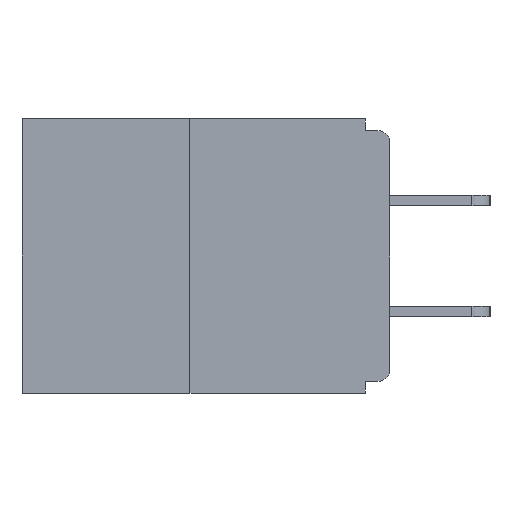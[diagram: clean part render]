
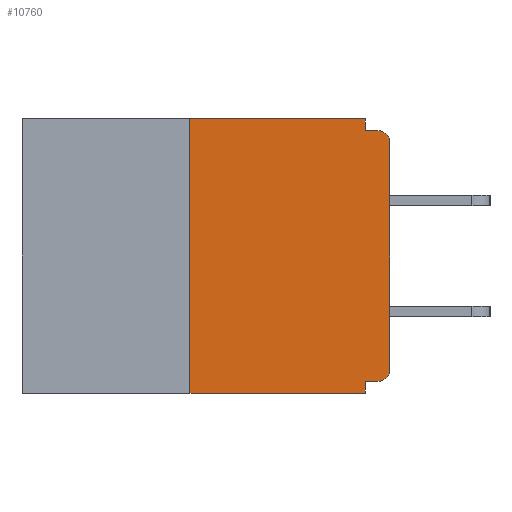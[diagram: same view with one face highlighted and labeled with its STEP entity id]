
A CAD part, left-side view. The second image highlights one B-rep face of the part: STEP entity #10760.
In plain terms, the highlighted planar face has unit normal (-1, 0, 0).
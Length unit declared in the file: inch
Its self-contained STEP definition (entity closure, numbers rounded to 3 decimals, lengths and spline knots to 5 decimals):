
#890 = LINE ( 'NONE', #17852, #12626 ) ;
#1479 = FACE_OUTER_BOUND ( 'NONE', #20674, .T. ) ;
#1658 = EDGE_CURVE ( 'NONE', #22780, #31343, #8278, .T. ) ;
#1729 = DIRECTION ( 'NONE',  ( 0., 0., -1. ) ) ;
#1784 = CARTESIAN_POINT ( 'NONE',  ( 0., 0.031, 0. ) ) ;
#2035 = DIRECTION ( 'NONE',  ( 0., 0., -1. ) ) ;
#2279 = AXIS2_PLACEMENT_3D ( 'NONE', #23241, #10829, #30538 ) ;
#2315 = VECTOR ( 'NONE', #21846, 39.37008 ) ;
#2624 = CARTESIAN_POINT ( 'NONE',  ( 0., 0.46, -0.343 ) ) ;
#2705 = CARTESIAN_POINT ( 'NONE',  ( 0., 0., -0.03 ) ) ;
#3207 = EDGE_CURVE ( 'NONE', #7098, #22780, #890, .T. ) ;
#3478 = LINE ( 'NONE', #25552, #4742 ) ;
#4213 = ORIENTED_EDGE ( 'NONE', *, *, #1658, .F. ) ;
#4228 = CARTESIAN_POINT ( 'NONE',  ( 0., 0.015, -0.03 ) ) ;
#4742 = VECTOR ( 'NONE', #1729, 39.37008 ) ;
#4753 = ORIENTED_EDGE ( 'NONE', *, *, #20375, .T. ) ;
#5220 = CARTESIAN_POINT ( 'NONE',  ( 0., 0.25, 0. ) ) ;
#5542 = CIRCLE ( 'NONE', #27365, 0.015 ) ;
#5695 = VECTOR ( 'NONE', #2035, 39.37008 ) ;
#6426 = DIRECTION ( 'NONE',  ( 0., 0., -1. ) ) ;
#6521 = CARTESIAN_POINT ( 'NONE',  ( 0., 0., -0.328 ) ) ;
#6990 = EDGE_CURVE ( 'NONE', #10298, #8557, #23359, .T. ) ;
#7098 = VERTEX_POINT ( 'NONE', #5220 ) ;
#7487 = EDGE_CURVE ( 'NONE', #10595, #27590, #17248, .T. ) ;
#7835 = CARTESIAN_POINT ( 'NONE',  ( 0., 0., -0.313 ) ) ;
#8038 = DIRECTION ( 'NONE',  ( 0., -1., 0. ) ) ;
#8278 = LINE ( 'NONE', #28575, #5695 ) ;
#8441 = VECTOR ( 'NONE', #30998, 39.37008 ) ;
#8557 = VERTEX_POINT ( 'NONE', #23411 ) ;
#9157 = DIRECTION ( 'NONE',  ( -1., 0., 0. ) ) ;
#9995 = ORIENTED_EDGE ( 'NONE', *, *, #3207, .F. ) ;
#10092 = EDGE_CURVE ( 'NONE', #31343, #21655, #12314, .T. ) ;
#10298 = VERTEX_POINT ( 'NONE', #30102 ) ;
#10595 = VERTEX_POINT ( 'NONE', #7835 ) ;
#10760 = ADVANCED_FACE ( 'NONE', ( #1479 ), #28008, .F. ) ;
#10829 = DIRECTION ( 'NONE',  ( 1., 0., 0. ) ) ;
#11262 = DIRECTION ( 'NONE',  ( 0., 1., 0. ) ) ;
#11376 = VECTOR ( 'NONE', #11262, 39.37008 ) ;
#12100 = ORIENTED_EDGE ( 'NONE', *, *, #17740, .F. ) ;
#12233 = CARTESIAN_POINT ( 'NONE',  ( 0., 0.25, 0. ) ) ;
#12314 = LINE ( 'NONE', #24564, #24607 ) ;
#12626 = VECTOR ( 'NONE', #29948, 39.37008 ) ;
#13742 = ORIENTED_EDGE ( 'NONE', *, *, #27082, .T. ) ;
#13960 = CIRCLE ( 'NONE', #22115, 0.015 ) ;
#15684 = ORIENTED_EDGE ( 'NONE', *, *, #25093, .F. ) ;
#17248 = LINE ( 'NONE', #17406, #26660 ) ;
#17309 = EDGE_CURVE ( 'NONE', #27590, #21655, #13960, .T. ) ;
#17359 = VERTEX_POINT ( 'NONE', #18833 ) ;
#17406 = CARTESIAN_POINT ( 'NONE',  ( 0., 0., 0. ) ) ;
#17740 = EDGE_CURVE ( 'NONE', #17359, #7098, #19546, .T. ) ;
#17852 = CARTESIAN_POINT ( 'NONE',  ( 0., 0.46, 0. ) ) ;
#18833 = CARTESIAN_POINT ( 'NONE',  ( 0., 0.25, -0.343 ) ) ;
#18901 = ORIENTED_EDGE ( 'NONE', *, *, #7487, .T. ) ;
#19546 = LINE ( 'NONE', #12233, #8441 ) ;
#20052 = ORIENTED_EDGE ( 'NONE', *, *, #17309, .T. ) ;
#20375 = EDGE_CURVE ( 'NONE', #10298, #10595, #5542, .T. ) ;
#20674 = EDGE_LOOP ( 'NONE', ( #9995, #12100, #13742, #15684, #28543, #4753, #18901, #20052, #26942, #4213 ) ) ;
#21655 = VERTEX_POINT ( 'NONE', #21822 ) ;
#21822 = CARTESIAN_POINT ( 'NONE',  ( 0., 0.015, -0.015 ) ) ;
#21846 = DIRECTION ( 'NONE',  ( 0., -1., 0. ) ) ;
#22115 = AXIS2_PLACEMENT_3D ( 'NONE', #4228, #9157, #30761 ) ;
#22780 = VERTEX_POINT ( 'NONE', #1784 ) ;
#23241 = CARTESIAN_POINT ( 'NONE',  ( 0., 0.46, 0. ) ) ;
#23269 = CARTESIAN_POINT ( 'NONE',  ( 0., 0.015, -0.313 ) ) ;
#23359 = LINE ( 'NONE', #6521, #11376 ) ;
#23411 = CARTESIAN_POINT ( 'NONE',  ( 0., 0.031, -0.328 ) ) ;
#24392 = LINE ( 'NONE', #2624, #2315 ) ;
#24564 = CARTESIAN_POINT ( 'NONE',  ( 0., 0., -0.015 ) ) ;
#24607 = VECTOR ( 'NONE', #8038, 39.37008 ) ;
#25093 = EDGE_CURVE ( 'NONE', #8557, #30930, #3478, .T. ) ;
#25552 = CARTESIAN_POINT ( 'NONE',  ( 0., 0.031, -0.343 ) ) ;
#26660 = VECTOR ( 'NONE', #27113, 39.37008 ) ;
#26731 = CARTESIAN_POINT ( 'NONE',  ( 0., 0.031, -0.015 ) ) ;
#26942 = ORIENTED_EDGE ( 'NONE', *, *, #10092, .F. ) ;
#27082 = EDGE_CURVE ( 'NONE', #17359, #30930, #24392, .T. ) ;
#27087 = CARTESIAN_POINT ( 'NONE',  ( 0., 0.031, -0.343 ) ) ;
#27113 = DIRECTION ( 'NONE',  ( 0., 0., 1. ) ) ;
#27365 = AXIS2_PLACEMENT_3D ( 'NONE', #23269, #28191, #6426 ) ;
#27590 = VERTEX_POINT ( 'NONE', #2705 ) ;
#28008 = PLANE ( 'NONE',  #2279 ) ;
#28191 = DIRECTION ( 'NONE',  ( -1., 0., 0. ) ) ;
#28543 = ORIENTED_EDGE ( 'NONE', *, *, #6990, .F. ) ;
#28575 = CARTESIAN_POINT ( 'NONE',  ( 0., 0.031, 0. ) ) ;
#29948 = DIRECTION ( 'NONE',  ( 0., -1., 0. ) ) ;
#30102 = CARTESIAN_POINT ( 'NONE',  ( 0., 0.015, -0.328 ) ) ;
#30538 = DIRECTION ( 'NONE',  ( 0., 0., -1. ) ) ;
#30761 = DIRECTION ( 'NONE',  ( 0., 0., -1. ) ) ;
#30930 = VERTEX_POINT ( 'NONE', #27087 ) ;
#30998 = DIRECTION ( 'NONE',  ( 0., 0., 1. ) ) ;
#31343 = VERTEX_POINT ( 'NONE', #26731 ) ;
